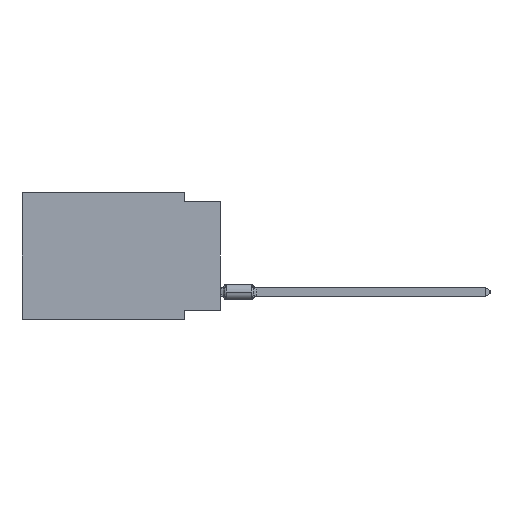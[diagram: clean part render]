
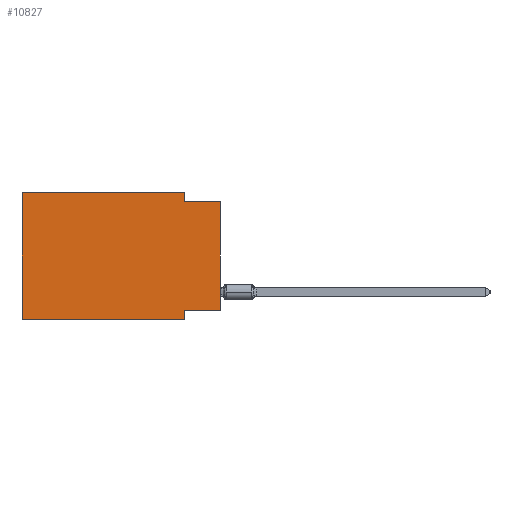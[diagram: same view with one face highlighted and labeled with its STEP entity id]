
A CAD part, left-side view. The second image highlights one B-rep face of the part: STEP entity #10827.
In plain terms, the highlighted planar face has unit normal (-1, 0, 0).
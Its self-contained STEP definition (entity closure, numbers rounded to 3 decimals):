
#159 = ORIENTED_EDGE ( 'NONE', *, *, #14491, .F. ) ;
#484 = CARTESIAN_POINT ( 'NONE',  ( 0., 13.97, -8.89 ) ) ;
#654 = ORIENTED_EDGE ( 'NONE', *, *, #24244, .T. ) ;
#739 = DIRECTION ( 'NONE',  ( 0., 0., -1. ) ) ;
#753 = EDGE_CURVE ( 'NONE', #13576, #22340, #1314, .T. ) ;
#1314 = LINE ( 'NONE', #13081, #29659 ) ;
#1654 = FACE_OUTER_BOUND ( 'NONE', #36784, .T. ) ;
#1888 = VECTOR ( 'NONE', #24032, 1000. ) ;
#4874 = ORIENTED_EDGE ( 'NONE', *, *, #10818, .F. ) ;
#5569 = DIRECTION ( 'NONE',  ( 0., -1., 0. ) ) ;
#5659 = VERTEX_POINT ( 'NONE', #12674 ) ;
#7084 = CARTESIAN_POINT ( 'NONE',  ( 0., 0., 0. ) ) ;
#7137 = VERTEX_POINT ( 'NONE', #30225 ) ;
#7328 = LINE ( 'NONE', #25084, #20133 ) ;
#10789 = LINE ( 'NONE', #28136, #37098 ) ;
#10818 = EDGE_CURVE ( 'NONE', #23933, #22179, #30992, .T. ) ;
#10827 = ADVANCED_FACE ( 'NONE', ( #1654 ), #13410, .F. ) ;
#11106 = ORIENTED_EDGE ( 'NONE', *, *, #24710, .F. ) ;
#11174 = VECTOR ( 'NONE', #739, 1000. ) ;
#11362 = ORIENTED_EDGE ( 'NONE', *, *, #25161, .F. ) ;
#11775 = VECTOR ( 'NONE', #28090, 1000. ) ;
#12158 = CARTESIAN_POINT ( 'NONE',  ( 0., 0., -0.635 ) ) ;
#12674 = CARTESIAN_POINT ( 'NONE',  ( 0., 13.97, 0. ) ) ;
#13081 = CARTESIAN_POINT ( 'NONE',  ( 0., 13.97, -8.89 ) ) ;
#13410 = PLANE ( 'NONE',  #32124 ) ;
#13576 = VERTEX_POINT ( 'NONE', #484 ) ;
#14093 = ORIENTED_EDGE ( 'NONE', *, *, #753, .T. ) ;
#14491 = EDGE_CURVE ( 'NONE', #5659, #15067, #7328, .T. ) ;
#15055 = VECTOR ( 'NONE', #5569, 1000. ) ;
#15067 = VERTEX_POINT ( 'NONE', #22890 ) ;
#15129 = LINE ( 'NONE', #30181, #17930 ) ;
#16326 = CARTESIAN_POINT ( 'NONE',  ( 0., 0., -8.255 ) ) ;
#16561 = DIRECTION ( 'NONE',  ( 0., 0., -1. ) ) ;
#17930 = VECTOR ( 'NONE', #20899, 1000. ) ;
#18493 = CARTESIAN_POINT ( 'NONE',  ( 0., 0., -8.255 ) ) ;
#19222 = CARTESIAN_POINT ( 'NONE',  ( 0., 2.54, -8.255 ) ) ;
#19606 = CARTESIAN_POINT ( 'NONE',  ( 0., 2.54, -8.89 ) ) ;
#20133 = VECTOR ( 'NONE', #22376, 1000. ) ;
#20899 = DIRECTION ( 'NONE',  ( 0., 0., 1. ) ) ;
#22179 = VERTEX_POINT ( 'NONE', #19222 ) ;
#22285 = DIRECTION ( 'NONE',  ( 1., 0., 0. ) ) ;
#22340 = VERTEX_POINT ( 'NONE', #19606 ) ;
#22376 = DIRECTION ( 'NONE',  ( 0., -1., 0. ) ) ;
#22890 = CARTESIAN_POINT ( 'NONE',  ( 0., 2.54, 0. ) ) ;
#23295 = CARTESIAN_POINT ( 'NONE',  ( 0., 0., -0.635 ) ) ;
#23933 = VERTEX_POINT ( 'NONE', #18493 ) ;
#24032 = DIRECTION ( 'NONE',  ( 0., 0., 1. ) ) ;
#24244 = EDGE_CURVE ( 'NONE', #23933, #30647, #27705, .T. ) ;
#24710 = EDGE_CURVE ( 'NONE', #13576, #5659, #15129, .T. ) ;
#25084 = CARTESIAN_POINT ( 'NONE',  ( 0., 13.97, 0. ) ) ;
#25161 = EDGE_CURVE ( 'NONE', #15067, #7137, #27739, .T. ) ;
#25183 = CARTESIAN_POINT ( 'NONE',  ( 0., 13.97, 0. ) ) ;
#25828 = ORIENTED_EDGE ( 'NONE', *, *, #36957, .F. ) ;
#27167 = CARTESIAN_POINT ( 'NONE',  ( 0., 2.54, 0. ) ) ;
#27705 = LINE ( 'NONE', #7084, #1888 ) ;
#27739 = LINE ( 'NONE', #27167, #11174 ) ;
#28090 = DIRECTION ( 'NONE',  ( 0., 1., 0. ) ) ;
#28136 = CARTESIAN_POINT ( 'NONE',  ( 0., 2.54, -8.89 ) ) ;
#29306 = LINE ( 'NONE', #23295, #15055 ) ;
#29659 = VECTOR ( 'NONE', #36663, 1000. ) ;
#30181 = CARTESIAN_POINT ( 'NONE',  ( 0., 13.97, 0. ) ) ;
#30225 = CARTESIAN_POINT ( 'NONE',  ( 0., 2.54, -0.635 ) ) ;
#30647 = VERTEX_POINT ( 'NONE', #12158 ) ;
#30879 = EDGE_CURVE ( 'NONE', #7137, #30647, #29306, .T. ) ;
#30992 = LINE ( 'NONE', #16326, #11775 ) ;
#32124 = AXIS2_PLACEMENT_3D ( 'NONE', #25183, #22285, #34080 ) ;
#34080 = DIRECTION ( 'NONE',  ( 0., 0., -1. ) ) ;
#34361 = ORIENTED_EDGE ( 'NONE', *, *, #30879, .F. ) ;
#36663 = DIRECTION ( 'NONE',  ( 0., -1., 0. ) ) ;
#36784 = EDGE_LOOP ( 'NONE', ( #654, #34361, #11362, #159, #11106, #14093, #25828, #4874 ) ) ;
#36957 = EDGE_CURVE ( 'NONE', #22179, #22340, #10789, .T. ) ;
#37098 = VECTOR ( 'NONE', #16561, 1000. ) ;
